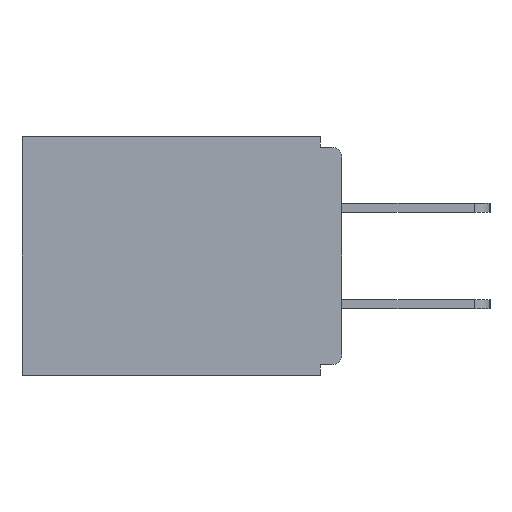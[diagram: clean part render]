
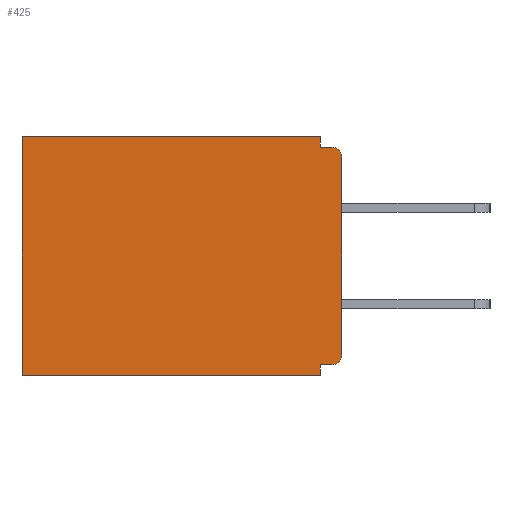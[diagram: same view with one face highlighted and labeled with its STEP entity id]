
A CAD part, left-side view. The second image highlights one B-rep face of the part: STEP entity #425.
In plain terms, the highlighted planar face has unit normal (-1, 0, 0).
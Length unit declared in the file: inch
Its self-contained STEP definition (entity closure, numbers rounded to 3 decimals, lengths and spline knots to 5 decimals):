
#119 = ORIENTED_EDGE ( 'NONE', *, *, #19014, .T. ) ;
#173 = ORIENTED_EDGE ( 'NONE', *, *, #14519, .F. ) ;
#425 = ADVANCED_FACE ( 'NONE', ( #4948 ), #9145, .F. ) ;
#761 = ORIENTED_EDGE ( 'NONE', *, *, #8639, .F. ) ;
#1181 = VERTEX_POINT ( 'NONE', #18444 ) ;
#1392 = DIRECTION ( 'NONE',  ( 0., -1., 0. ) ) ;
#1571 = CARTESIAN_POINT ( 'NONE',  ( 0.298, 0., 0. ) ) ;
#1759 = EDGE_CURVE ( 'NONE', #1181, #3796, #16988, .T. ) ;
#1828 = DIRECTION ( 'NONE',  ( 0., 0., -1. ) ) ;
#2105 = CARTESIAN_POINT ( 'NONE',  ( 0.298, 0.031, -0.328 ) ) ;
#2121 = DIRECTION ( 'NONE',  ( -1., 0., 0. ) ) ;
#2573 = CARTESIAN_POINT ( 'NONE',  ( 0.298, 0.46, -0.343 ) ) ;
#2942 = AXIS2_PLACEMENT_3D ( 'NONE', #5129, #2121, #17512 ) ;
#3033 = VECTOR ( 'NONE', #5406, 39.37008 ) ;
#3125 = CARTESIAN_POINT ( 'NONE',  ( 0.298, 0., -0.343 ) ) ;
#3201 = DIRECTION ( 'NONE',  ( 0., 0., -1. ) ) ;
#3523 = LINE ( 'NONE', #8598, #3033 ) ;
#3572 = DIRECTION ( 'NONE',  ( 0., 1., 0. ) ) ;
#3672 = DIRECTION ( 'NONE',  ( 0., 1., 0. ) ) ;
#3761 = VECTOR ( 'NONE', #1392, 39.37008 ) ;
#3796 = VERTEX_POINT ( 'NONE', #17833 ) ;
#4279 = CARTESIAN_POINT ( 'NONE',  ( 0.298, 0., -0.015 ) ) ;
#4588 = VERTEX_POINT ( 'NONE', #18315 ) ;
#4616 = VERTEX_POINT ( 'NONE', #6920 ) ;
#4895 = CARTESIAN_POINT ( 'NONE',  ( 0.298, 0.031, -0.343 ) ) ;
#4948 = FACE_OUTER_BOUND ( 'NONE', #18402, .T. ) ;
#5129 = CARTESIAN_POINT ( 'NONE',  ( 0.298, 0.015, -0.03 ) ) ;
#5307 = LINE ( 'NONE', #5717, #17655 ) ;
#5406 = DIRECTION ( 'NONE',  ( 0., 0., -1. ) ) ;
#5717 = CARTESIAN_POINT ( 'NONE',  ( 0.298, 0.46, 0. ) ) ;
#5779 = DIRECTION ( 'NONE',  ( 0., 0., -1. ) ) ;
#5819 = EDGE_CURVE ( 'NONE', #12364, #18017, #3523, .T. ) ;
#6488 = ORIENTED_EDGE ( 'NONE', *, *, #15580, .F. ) ;
#6544 = CARTESIAN_POINT ( 'NONE',  ( 0.298, 0.015, -0.313 ) ) ;
#6920 = CARTESIAN_POINT ( 'NONE',  ( 0.298, 0.031, -0.343 ) ) ;
#7799 = VECTOR ( 'NONE', #16489, 39.37008 ) ;
#7900 = VECTOR ( 'NONE', #3572, 39.37008 ) ;
#8436 = CARTESIAN_POINT ( 'NONE',  ( 0.298, 0.015, -0.015 ) ) ;
#8598 = CARTESIAN_POINT ( 'NONE',  ( 0.298, 0.031, -0.343 ) ) ;
#8639 = EDGE_CURVE ( 'NONE', #8725, #4616, #9738, .T. ) ;
#8725 = VERTEX_POINT ( 'NONE', #2105 ) ;
#8912 = EDGE_CURVE ( 'NONE', #12364, #4588, #11466, .T. ) ;
#9136 = ORIENTED_EDGE ( 'NONE', *, *, #5819, .F. ) ;
#9145 = PLANE ( 'NONE',  #14370 ) ;
#9536 = VERTEX_POINT ( 'NONE', #2573 ) ;
#9738 = LINE ( 'NONE', #4895, #19169 ) ;
#9753 = EDGE_CURVE ( 'NONE', #1181, #16996, #18651, .T. ) ;
#9904 = ORIENTED_EDGE ( 'NONE', *, *, #1759, .F. ) ;
#11466 = LINE ( 'NONE', #11907, #7799 ) ;
#11907 = CARTESIAN_POINT ( 'NONE',  ( 0.298, 0., 0. ) ) ;
#11940 = CARTESIAN_POINT ( 'NONE',  ( 0.298, 0.031, -0.015 ) ) ;
#12213 = ORIENTED_EDGE ( 'NONE', *, *, #8912, .T. ) ;
#12364 = VERTEX_POINT ( 'NONE', #15943 ) ;
#12451 = VECTOR ( 'NONE', #3672, 39.37008 ) ;
#12458 = DIRECTION ( 'NONE',  ( 0., 0., -1. ) ) ;
#12578 = DIRECTION ( 'NONE',  ( -1., 0., 0. ) ) ;
#12675 = EDGE_CURVE ( 'NONE', #18017, #16996, #15890, .T. ) ;
#13242 = LINE ( 'NONE', #19113, #7900 ) ;
#13271 = ORIENTED_EDGE ( 'NONE', *, *, #9753, .T. ) ;
#13883 = CARTESIAN_POINT ( 'NONE',  ( 0.298, 0., 0. ) ) ;
#13947 = DIRECTION ( 'NONE',  ( 1., 0., 0. ) ) ;
#14010 = ORIENTED_EDGE ( 'NONE', *, *, #12675, .F. ) ;
#14370 = AXIS2_PLACEMENT_3D ( 'NONE', #13883, #13947, #16922 ) ;
#14519 = EDGE_CURVE ( 'NONE', #18406, #8725, #13242, .T. ) ;
#15580 = EDGE_CURVE ( 'NONE', #4616, #9536, #18026, .T. ) ;
#15890 = LINE ( 'NONE', #4279, #3761 ) ;
#15943 = CARTESIAN_POINT ( 'NONE',  ( 0.298, 0.031, 0. ) ) ;
#16489 = DIRECTION ( 'NONE',  ( 0., 1., 0. ) ) ;
#16922 = DIRECTION ( 'NONE',  ( 0., 0., -1. ) ) ;
#16988 = LINE ( 'NONE', #1571, #18202 ) ;
#16996 = VERTEX_POINT ( 'NONE', #8436 ) ;
#17512 = DIRECTION ( 'NONE',  ( 0., 0., -1. ) ) ;
#17655 = VECTOR ( 'NONE', #5779, 39.37008 ) ;
#17833 = CARTESIAN_POINT ( 'NONE',  ( 0.298, 0., -0.313 ) ) ;
#17860 = CARTESIAN_POINT ( 'NONE',  ( 0.298, 0.015, -0.328 ) ) ;
#18017 = VERTEX_POINT ( 'NONE', #11940 ) ;
#18026 = LINE ( 'NONE', #3125, #12451 ) ;
#18202 = VECTOR ( 'NONE', #12458, 39.37008 ) ;
#18218 = ORIENTED_EDGE ( 'NONE', *, *, #19337, .T. ) ;
#18315 = CARTESIAN_POINT ( 'NONE',  ( 0.298, 0.46, 0. ) ) ;
#18402 = EDGE_LOOP ( 'NONE', ( #13271, #14010, #9136, #12213, #119, #6488, #761, #173, #18218, #9904 ) ) ;
#18406 = VERTEX_POINT ( 'NONE', #17860 ) ;
#18444 = CARTESIAN_POINT ( 'NONE',  ( 0.298, 0., -0.03 ) ) ;
#18651 = CIRCLE ( 'NONE', #2942, 0.015 ) ;
#18665 = AXIS2_PLACEMENT_3D ( 'NONE', #6544, #12578, #3201 ) ;
#19014 = EDGE_CURVE ( 'NONE', #4588, #9536, #5307, .T. ) ;
#19113 = CARTESIAN_POINT ( 'NONE',  ( 0.298, 0., -0.328 ) ) ;
#19169 = VECTOR ( 'NONE', #1828, 39.37008 ) ;
#19337 = EDGE_CURVE ( 'NONE', #18406, #3796, #19571, .T. ) ;
#19571 = CIRCLE ( 'NONE', #18665, 0.015 ) ;
